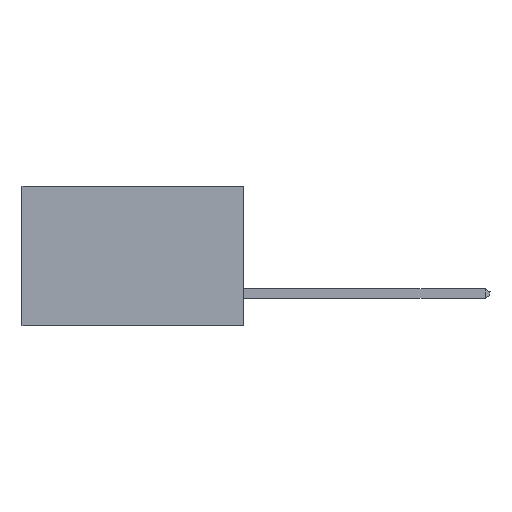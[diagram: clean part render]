
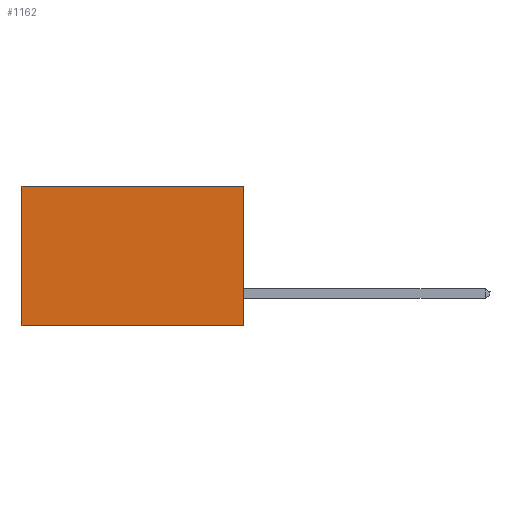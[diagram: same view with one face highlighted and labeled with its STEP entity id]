
A CAD part, left-side view. The second image highlights one B-rep face of the part: STEP entity #1162.
In plain terms, the highlighted planar face has unit normal (-1, 0, 0).
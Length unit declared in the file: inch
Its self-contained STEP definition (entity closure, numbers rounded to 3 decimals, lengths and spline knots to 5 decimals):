
#31 = ORIENTED_EDGE ( 'NONE', *, *, #12592, .F. ) ;
#1084 = FACE_OUTER_BOUND ( 'NONE', #11827, .T. ) ;
#1162 = ADVANCED_FACE ( 'NONE', ( #1084 ), #1628, .F. ) ;
#1422 = VERTEX_POINT ( 'NONE', #5933 ) ;
#1628 = PLANE ( 'NONE',  #13808 ) ;
#1711 = CARTESIAN_POINT ( 'NONE',  ( 0.277, 0., -0.37 ) ) ;
#1748 = CARTESIAN_POINT ( 'NONE',  ( 0.277, 0.59, 0. ) ) ;
#1814 = VECTOR ( 'NONE', #12439, 39.37008 ) ;
#2110 = DIRECTION ( 'NONE',  ( 1., 0., 0. ) ) ;
#2805 = ORIENTED_EDGE ( 'NONE', *, *, #7083, .T. ) ;
#3057 = DIRECTION ( 'NONE',  ( 0., 0., -1. ) ) ;
#3139 = VERTEX_POINT ( 'NONE', #9817 ) ;
#3603 = CARTESIAN_POINT ( 'NONE',  ( 0.277, 0., -0.37 ) ) ;
#4331 = ORIENTED_EDGE ( 'NONE', *, *, #4943, .F. ) ;
#4943 = EDGE_CURVE ( 'NONE', #3139, #6248, #12387, .T. ) ;
#5276 = CARTESIAN_POINT ( 'NONE',  ( 0.277, 0., -0.37 ) ) ;
#5716 = CARTESIAN_POINT ( 'NONE',  ( 0.277, 0., -0.37 ) ) ;
#5933 = CARTESIAN_POINT ( 'NONE',  ( 0.277, 0.59, -0.37 ) ) ;
#6248 = VERTEX_POINT ( 'NONE', #3603 ) ;
#6293 = LINE ( 'NONE', #11023, #16348 ) ;
#6444 = LINE ( 'NONE', #13426, #9561 ) ;
#6708 = DIRECTION ( 'NONE',  ( 0., 0., -1. ) ) ;
#7083 = EDGE_CURVE ( 'NONE', #3139, #7861, #6444, .T. ) ;
#7704 = DIRECTION ( 'NONE',  ( 0., 1., 0. ) ) ;
#7861 = VERTEX_POINT ( 'NONE', #1748 ) ;
#9561 = VECTOR ( 'NONE', #7704, 39.37008 ) ;
#9817 = CARTESIAN_POINT ( 'NONE',  ( 0.277, 0., 0. ) ) ;
#11023 = CARTESIAN_POINT ( 'NONE',  ( 0.277, 0.59, -0.37 ) ) ;
#11261 = ORIENTED_EDGE ( 'NONE', *, *, #16133, .T. ) ;
#11827 = EDGE_LOOP ( 'NONE', ( #11261, #31, #4331, #2805 ) ) ;
#12243 = LINE ( 'NONE', #5276, #15649 ) ;
#12387 = LINE ( 'NONE', #5716, #1814 ) ;
#12439 = DIRECTION ( 'NONE',  ( 0., 0., -1. ) ) ;
#12592 = EDGE_CURVE ( 'NONE', #6248, #1422, #12243, .T. ) ;
#13426 = CARTESIAN_POINT ( 'NONE',  ( 0.277, 0., 0. ) ) ;
#13808 = AXIS2_PLACEMENT_3D ( 'NONE', #1711, #2110, #6708 ) ;
#14547 = DIRECTION ( 'NONE',  ( 0., 1., 0. ) ) ;
#15649 = VECTOR ( 'NONE', #14547, 39.37008 ) ;
#16133 = EDGE_CURVE ( 'NONE', #7861, #1422, #6293, .T. ) ;
#16348 = VECTOR ( 'NONE', #3057, 39.37008 ) ;
